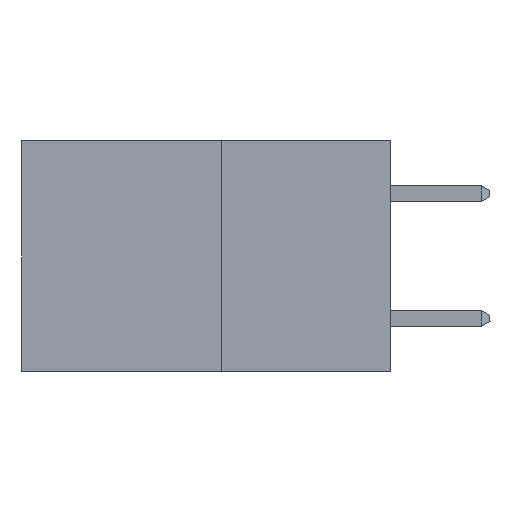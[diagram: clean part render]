
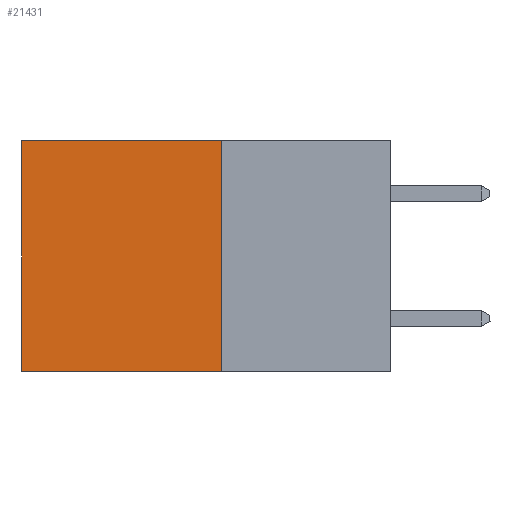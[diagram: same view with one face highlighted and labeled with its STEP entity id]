
A CAD part, left-side view. The second image highlights one B-rep face of the part: STEP entity #21431.
In plain terms, the highlighted planar face has unit normal (-1, 0, 0).
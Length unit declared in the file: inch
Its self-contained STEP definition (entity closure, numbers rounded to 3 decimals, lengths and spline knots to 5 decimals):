
#242 = LINE ( 'NONE', #17087, #4454 ) ;
#1140 = LINE ( 'NONE', #7870, #2289 ) ;
#1297 = CARTESIAN_POINT ( 'NONE',  ( 0.277, 0.27, -0.37 ) ) ;
#1407 = CARTESIAN_POINT ( 'NONE',  ( 0.277, 0.27, -0.37 ) ) ;
#1878 = ORIENTED_EDGE ( 'NONE', *, *, #22551, .F. ) ;
#2289 = VECTOR ( 'NONE', #14894, 39.37008 ) ;
#3149 = CARTESIAN_POINT ( 'NONE',  ( 0.277, 0.27, 0. ) ) ;
#3494 = ORIENTED_EDGE ( 'NONE', *, *, #19613, .T. ) ;
#3701 = VERTEX_POINT ( 'NONE', #14381 ) ;
#4454 = VECTOR ( 'NONE', #8233, 39.37008 ) ;
#6673 = AXIS2_PLACEMENT_3D ( 'NONE', #20832, #6741, #19124 ) ;
#6741 = DIRECTION ( 'NONE',  ( 1., 0., 0. ) ) ;
#6806 = VECTOR ( 'NONE', #19085, 39.37008 ) ;
#7323 = ORIENTED_EDGE ( 'NONE', *, *, #16382, .F. ) ;
#7870 = CARTESIAN_POINT ( 'NONE',  ( 0.277, 0.59, -0.37 ) ) ;
#8233 = DIRECTION ( 'NONE',  ( 0., 1., 0. ) ) ;
#10372 = VECTOR ( 'NONE', #17353, 39.37008 ) ;
#10932 = LINE ( 'NONE', #3149, #10372 ) ;
#11446 = LINE ( 'NONE', #1297, #6806 ) ;
#11591 = ORIENTED_EDGE ( 'NONE', *, *, #21881, .T. ) ;
#14381 = CARTESIAN_POINT ( 'NONE',  ( 0.277, 0.27, 0. ) ) ;
#14894 = DIRECTION ( 'NONE',  ( 0., 0., -1. ) ) ;
#15348 = FACE_OUTER_BOUND ( 'NONE', #16210, .T. ) ;
#15506 = CARTESIAN_POINT ( 'NONE',  ( 0.277, 0.59, -0.37 ) ) ;
#15718 = VERTEX_POINT ( 'NONE', #1407 ) ;
#16108 = CARTESIAN_POINT ( 'NONE',  ( 0.277, 0.59, 0. ) ) ;
#16210 = EDGE_LOOP ( 'NONE', ( #11591, #1878, #7323, #3494 ) ) ;
#16382 = EDGE_CURVE ( 'NONE', #3701, #15718, #11446, .T. ) ;
#17087 = CARTESIAN_POINT ( 'NONE',  ( 0.277, 0.27, -0.37 ) ) ;
#17341 = VERTEX_POINT ( 'NONE', #16108 ) ;
#17353 = DIRECTION ( 'NONE',  ( 0., 1., 0. ) ) ;
#17363 = PLANE ( 'NONE',  #6673 ) ;
#18332 = VERTEX_POINT ( 'NONE', #15506 ) ;
#19085 = DIRECTION ( 'NONE',  ( 0., 0., -1. ) ) ;
#19124 = DIRECTION ( 'NONE',  ( 0., 0., -1. ) ) ;
#19613 = EDGE_CURVE ( 'NONE', #3701, #17341, #10932, .T. ) ;
#20832 = CARTESIAN_POINT ( 'NONE',  ( 0.277, 0.27, -0.37 ) ) ;
#21431 = ADVANCED_FACE ( 'NONE', ( #15348 ), #17363, .F. ) ;
#21881 = EDGE_CURVE ( 'NONE', #17341, #18332, #1140, .T. ) ;
#22551 = EDGE_CURVE ( 'NONE', #15718, #18332, #242, .T. ) ;
